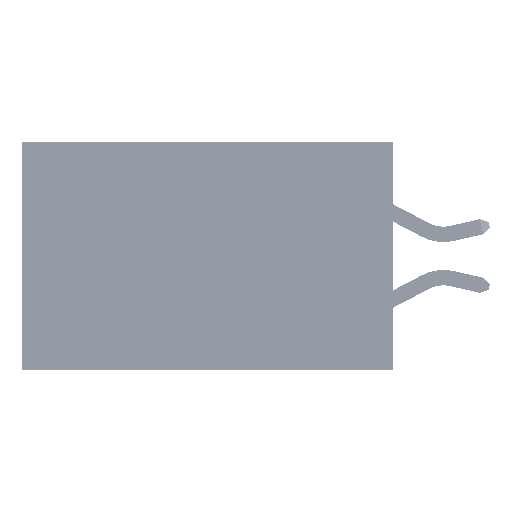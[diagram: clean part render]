
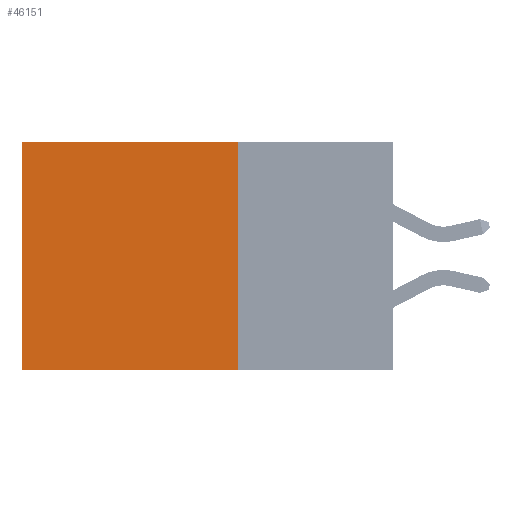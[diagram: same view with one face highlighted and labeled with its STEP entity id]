
A CAD part, left-side view. The second image highlights one B-rep face of the part: STEP entity #46151.
In plain terms, the highlighted planar face has unit normal (-1, 0, 0).
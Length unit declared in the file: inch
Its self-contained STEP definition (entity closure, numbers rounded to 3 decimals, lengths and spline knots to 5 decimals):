
#797 = CARTESIAN_POINT ( 'NONE',  ( 0.2875, 0.25, -0.37 ) ) ;
#3661 = CARTESIAN_POINT ( 'NONE',  ( 0.2875, 0.25, 0. ) ) ;
#4953 = CARTESIAN_POINT ( 'NONE',  ( 0.2875, 0.25, 0. ) ) ;
#6844 = DIRECTION ( 'NONE',  ( 0., 1., 0. ) ) ;
#8281 = CARTESIAN_POINT ( 'NONE',  ( 0.2875, 0.6, 0. ) ) ;
#8963 = PLANE ( 'NONE',  #41270 ) ;
#14455 = ORIENTED_EDGE ( 'NONE', *, *, #20475, .F. ) ;
#16427 = EDGE_CURVE ( 'NONE', #16500, #48523, #27713, .T. ) ;
#16500 = VERTEX_POINT ( 'NONE', #19854 ) ;
#16892 = EDGE_CURVE ( 'NONE', #47950, #41483, #38164, .T. ) ;
#17084 = VECTOR ( 'NONE', #35970, 39.37008 ) ;
#19854 = CARTESIAN_POINT ( 'NONE',  ( 0.2875, 0.25, 0. ) ) ;
#20475 = EDGE_CURVE ( 'NONE', #48523, #41483, #31701, .T. ) ;
#21405 = VECTOR ( 'NONE', #29742, 39.37008 ) ;
#27713 = LINE ( 'NONE', #3661, #17084 ) ;
#29742 = DIRECTION ( 'NONE',  ( 0., 0., -1. ) ) ;
#30526 = FACE_OUTER_BOUND ( 'NONE', #33871, .T. ) ;
#31701 = LINE ( 'NONE', #797, #47761 ) ;
#31910 = LINE ( 'NONE', #38461, #32502 ) ;
#32502 = VECTOR ( 'NONE', #6844, 39.37008 ) ;
#33871 = EDGE_LOOP ( 'NONE', ( #43595, #14455, #39998, #35437 ) ) ;
#35068 = CARTESIAN_POINT ( 'NONE',  ( 0.2875, 0.25, -0.37 ) ) ;
#35437 = ORIENTED_EDGE ( 'NONE', *, *, #45089, .T. ) ;
#35970 = DIRECTION ( 'NONE',  ( 0., 0., -1. ) ) ;
#36703 = CARTESIAN_POINT ( 'NONE',  ( 0.2875, 0.6, 0. ) ) ;
#38164 = LINE ( 'NONE', #36703, #21405 ) ;
#38461 = CARTESIAN_POINT ( 'NONE',  ( 0.2875, 0.25, 0. ) ) ;
#39998 = ORIENTED_EDGE ( 'NONE', *, *, #16427, .F. ) ;
#41176 = CARTESIAN_POINT ( 'NONE',  ( 0.2875, 0.6, -0.37 ) ) ;
#41270 = AXIS2_PLACEMENT_3D ( 'NONE', #4953, #44500, #44841 ) ;
#41483 = VERTEX_POINT ( 'NONE', #41176 ) ;
#43595 = ORIENTED_EDGE ( 'NONE', *, *, #16892, .T. ) ;
#44342 = DIRECTION ( 'NONE',  ( 0., 1., 0. ) ) ;
#44500 = DIRECTION ( 'NONE',  ( 1., 0., 0. ) ) ;
#44841 = DIRECTION ( 'NONE',  ( 0., 0., -1. ) ) ;
#45089 = EDGE_CURVE ( 'NONE', #16500, #47950, #31910, .T. ) ;
#46151 = ADVANCED_FACE ( 'NONE', ( #30526 ), #8963, .F. ) ;
#47761 = VECTOR ( 'NONE', #44342, 39.37008 ) ;
#47950 = VERTEX_POINT ( 'NONE', #8281 ) ;
#48523 = VERTEX_POINT ( 'NONE', #35068 ) ;
